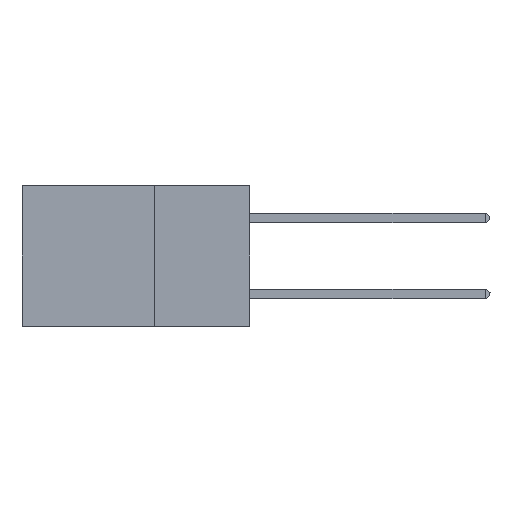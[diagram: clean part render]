
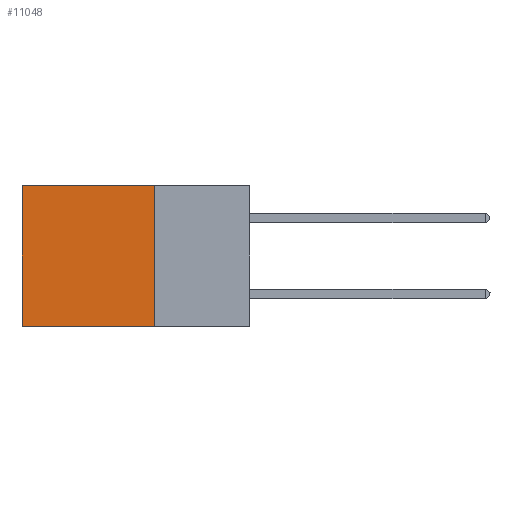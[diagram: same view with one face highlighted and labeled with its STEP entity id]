
A CAD part, left-side view. The second image highlights one B-rep face of the part: STEP entity #11048.
In plain terms, the highlighted planar face has unit normal (-1, 0, 0).
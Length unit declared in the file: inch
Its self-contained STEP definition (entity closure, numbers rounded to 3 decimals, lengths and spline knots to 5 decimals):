
#7 = VERTEX_POINT ( 'NONE', #5337 ) ;
#187 = DIRECTION ( 'NONE',  ( 0., 0., -1. ) ) ;
#591 = EDGE_LOOP ( 'NONE', ( #15860, #15124, #19504, #8051 ) ) ;
#1167 = EDGE_CURVE ( 'NONE', #5532, #7, #2651, .T. ) ;
#2651 = LINE ( 'NONE', #2873, #19649 ) ;
#2873 = CARTESIAN_POINT ( 'NONE',  ( 0.2875, 0.6, 0. ) ) ;
#3814 = LINE ( 'NONE', #8798, #18274 ) ;
#4276 = EDGE_CURVE ( 'NONE', #11289, #5532, #7908, .T. ) ;
#4506 = DIRECTION ( 'NONE',  ( 0., 1., 0. ) ) ;
#5337 = CARTESIAN_POINT ( 'NONE',  ( 0.2875, 0.6, -0.37 ) ) ;
#5532 = VERTEX_POINT ( 'NONE', #14620 ) ;
#5709 = VECTOR ( 'NONE', #16124, 39.37008 ) ;
#7086 = FACE_OUTER_BOUND ( 'NONE', #591, .T. ) ;
#7692 = CARTESIAN_POINT ( 'NONE',  ( 0.2875, 0.25, 0. ) ) ;
#7908 = LINE ( 'NONE', #7692, #14195 ) ;
#8051 = ORIENTED_EDGE ( 'NONE', *, *, #4276, .T. ) ;
#8087 = CARTESIAN_POINT ( 'NONE',  ( 0.2875, 0.25, 0. ) ) ;
#8684 = CARTESIAN_POINT ( 'NONE',  ( 0.2875, 0.25, 0. ) ) ;
#8798 = CARTESIAN_POINT ( 'NONE',  ( 0.2875, 0.25, 0. ) ) ;
#9215 = CARTESIAN_POINT ( 'NONE',  ( 0.2875, 0.25, -0.37 ) ) ;
#11048 = ADVANCED_FACE ( 'NONE', ( #7086 ), #12430, .F. ) ;
#11289 = VERTEX_POINT ( 'NONE', #8087 ) ;
#12098 = VERTEX_POINT ( 'NONE', #18996 ) ;
#12121 = EDGE_CURVE ( 'NONE', #11289, #12098, #3814, .T. ) ;
#12430 = PLANE ( 'NONE',  #17897 ) ;
#13780 = DIRECTION ( 'NONE',  ( 0., 0., -1. ) ) ;
#14195 = VECTOR ( 'NONE', #4506, 39.37008 ) ;
#14620 = CARTESIAN_POINT ( 'NONE',  ( 0.2875, 0.6, 0. ) ) ;
#15097 = DIRECTION ( 'NONE',  ( 0., 0., -1. ) ) ;
#15124 = ORIENTED_EDGE ( 'NONE', *, *, #16988, .F. ) ;
#15585 = DIRECTION ( 'NONE',  ( 1., 0., 0. ) ) ;
#15860 = ORIENTED_EDGE ( 'NONE', *, *, #1167, .T. ) ;
#16124 = DIRECTION ( 'NONE',  ( 0., 1., 0. ) ) ;
#16988 = EDGE_CURVE ( 'NONE', #12098, #7, #19959, .T. ) ;
#17897 = AXIS2_PLACEMENT_3D ( 'NONE', #8684, #15585, #13780 ) ;
#18274 = VECTOR ( 'NONE', #187, 39.37008 ) ;
#18996 = CARTESIAN_POINT ( 'NONE',  ( 0.2875, 0.25, -0.37 ) ) ;
#19504 = ORIENTED_EDGE ( 'NONE', *, *, #12121, .F. ) ;
#19649 = VECTOR ( 'NONE', #15097, 39.37008 ) ;
#19959 = LINE ( 'NONE', #9215, #5709 ) ;
